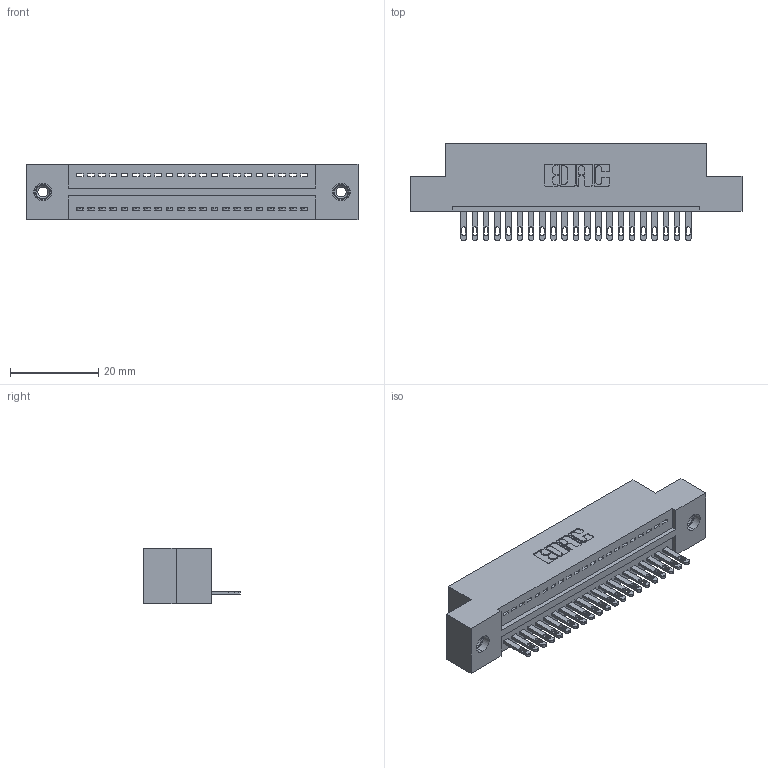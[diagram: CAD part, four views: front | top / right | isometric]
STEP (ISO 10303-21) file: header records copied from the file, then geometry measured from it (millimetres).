
FILE_DESCRIPTION (( 'STEP AP203' ), '1' );
FILE_NAME ('325-021-500-108.STEP', '2020-02-24T17:12:21', ( '' ), ( '' ), 'SwSTEP 2.0', 'SolidWorks 2016', '' );
FILE_SCHEMA (( 'CONFIG_CONTROL_DESIGN' ));
Length unit declared in the file: inch
Products named in the file (4): 325-021-500-108; 325 Part_TI; 345-250-001_345-250-003-102; 325-292-001_325-293-100
Assembly tree (24 placements, depth 2):
  325-021-500-108
    325 Part_TI
    325-292-001_325-293-100  x21
    345-250-001_345-250-003-102  x2
Bounding box: 75.06 x 21.84 x 12.45 mm (x, y, z)
Volume: 9369.9 mm3; surface area: 9944.9 mm2
Topology: 24 solids, 24 shells, 1308 faces, 3975 edges, 2642 vertices
Faces by surface type: plane 858, cylinder 434, cone 12, torus 4
Entity records: 16670 total; most frequent: CARTESIAN_POINT 2860, ORIENTED_EDGE 2810, DIRECTION 2489, EDGE_CURVE 1405, LINE 1253, VECTOR 1253, VERTEX_POINT 932, AXIS2_PLACEMENT_3D 618
